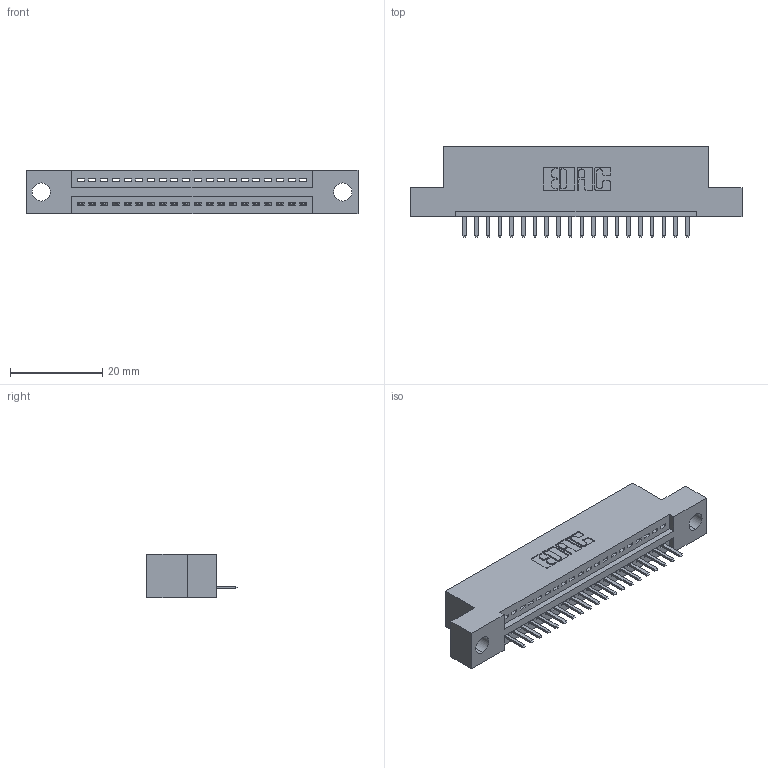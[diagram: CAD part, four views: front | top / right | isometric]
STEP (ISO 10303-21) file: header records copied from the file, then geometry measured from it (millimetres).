
FILE_DESCRIPTION (( 'STEP AP203' ), '1' );
FILE_NAME ('395-020-520-104.STEP', '2018-11-07T14:23:17', ( '' ), ( '' ), 'SwSTEP 2.0', 'SolidWorks 2016', '' );
FILE_SCHEMA (( 'CONFIG_CONTROL_DESIGN' ));
Length unit declared in the file: inch
Products named in the file (3): 395-020-520-104; 345-292-001_345-293-120; 345 Part_Flush Mounting Lugs - 0.156 Dia-TH
Assembly tree (21 placements, depth 2):
  395-020-520-104
    345 Part_Flush Mounting Lugs - 0.156 Dia-TH
    345-292-001_345-293-120  x20
Bounding box: 72.01 x 19.68 x 9.4 mm (x, y, z)
Volume: 6513.9 mm3; surface area: 7977.9 mm2
Topology: 21 solids, 21 shells, 1366 faces, 4021 edges, 2626 vertices
Faces by surface type: plane 920, cylinder 446
Entity records: 18131 total; most frequent: CARTESIAN_POINT 3160, ORIENTED_EDGE 3102, DIRECTION 2779, EDGE_CURVE 1551, LINE 1335, VECTOR 1335, VERTEX_POINT 1030, AXIS2_PLACEMENT_3D 722
